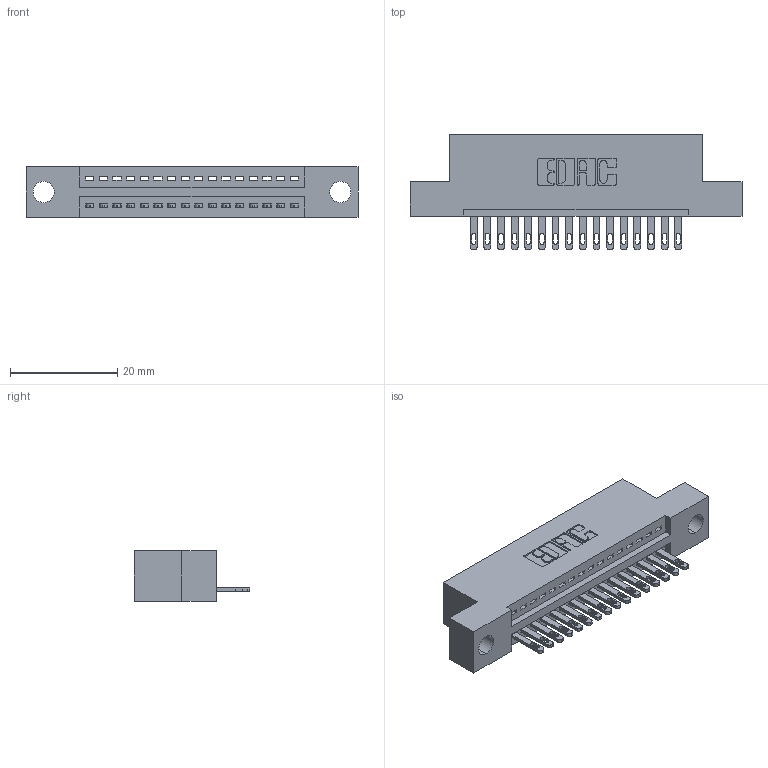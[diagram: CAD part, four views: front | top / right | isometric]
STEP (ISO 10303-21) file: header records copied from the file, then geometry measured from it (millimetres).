
FILE_DESCRIPTION (( 'STEP AP203' ), '1' );
FILE_NAME ('345-016-500-104.STEP', '2019-10-04T12:58:10', ( '' ), ( '' ), 'SwSTEP 2.0', 'SolidWorks 2016', '' );
FILE_SCHEMA (( 'CONFIG_CONTROL_DESIGN' ));
Length unit declared in the file: inch
Products named in the file (3): 345-016-500-104; 345-292-001_345-293-100; 345 Part_Flush Mounting Lugs - 0.156 Dia-TH
Assembly tree (17 placements, depth 2):
  345-016-500-104
    345 Part_Flush Mounting Lugs - 0.156 Dia-TH
    345-292-001_345-293-100  x16
Bounding box: 61.85 x 21.51 x 9.4 mm (x, y, z)
Volume: 5583.5 mm3; surface area: 6911.3 mm2
Topology: 17 solids, 17 shells, 990 faces, 3029 edges, 2018 vertices
Faces by surface type: plane 624, cylinder 366
Entity records: 15475 total; most frequent: CARTESIAN_POINT 2688, ORIENTED_EDGE 2638, DIRECTION 2387, EDGE_CURVE 1319, LINE 1119, VECTOR 1119, VERTEX_POINT 878, AXIS2_PLACEMENT_3D 634
